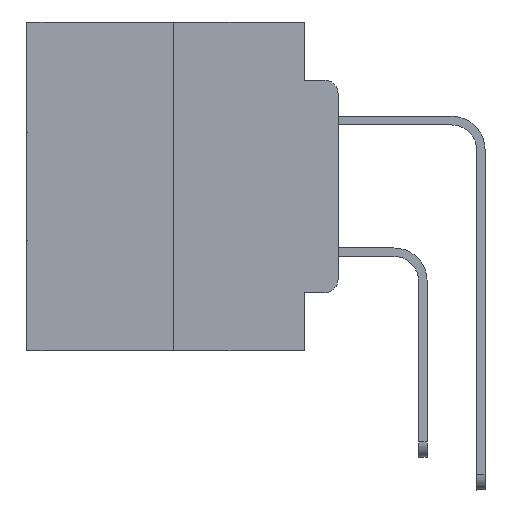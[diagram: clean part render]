
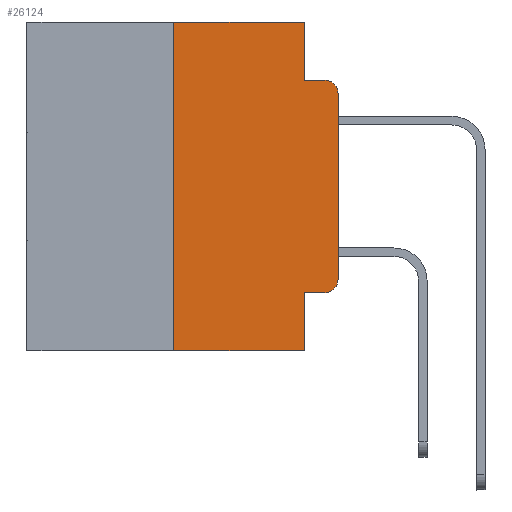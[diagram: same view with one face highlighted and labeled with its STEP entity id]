
A CAD part, left-side view. The second image highlights one B-rep face of the part: STEP entity #26124.
In plain terms, the highlighted planar face has unit normal (-1, 0, 0).
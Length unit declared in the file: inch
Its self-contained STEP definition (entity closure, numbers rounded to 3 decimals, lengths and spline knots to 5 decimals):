
#1481 = EDGE_CURVE ( 'NONE', #4113, #3315, #22992, .T. ) ;
#1578 = LINE ( 'NONE', #7016, #3726 ) ;
#1732 = DIRECTION ( 'NONE',  ( 1., 0., 0. ) ) ;
#2211 = VERTEX_POINT ( 'NONE', #15602 ) ;
#3315 = VERTEX_POINT ( 'NONE', #21942 ) ;
#3334 = ORIENTED_EDGE ( 'NONE', *, *, #27050, .T. ) ;
#3726 = VECTOR ( 'NONE', #4649, 39.37008 ) ;
#4071 = VECTOR ( 'NONE', #12313, 39.37008 ) ;
#4113 = VERTEX_POINT ( 'NONE', #10780 ) ;
#4649 = DIRECTION ( 'NONE',  ( 0., -1., 0. ) ) ;
#5080 = EDGE_CURVE ( 'NONE', #3315, #6023, #9863, .T. ) ;
#5183 = DIRECTION ( 'NONE',  ( -1., 0., 0. ) ) ;
#5289 = VERTEX_POINT ( 'NONE', #11602 ) ;
#6023 = VERTEX_POINT ( 'NONE', #20950 ) ;
#6051 = VERTEX_POINT ( 'NONE', #8245 ) ;
#6160 = PLANE ( 'NONE',  #24197 ) ;
#6342 = CARTESIAN_POINT ( 'NONE',  ( 0., 0.02, -0.0885 ) ) ;
#7016 = CARTESIAN_POINT ( 'NONE',  ( 0., 0.051, -0.0885 ) ) ;
#7912 = ORIENTED_EDGE ( 'NONE', *, *, #14384, .F. ) ;
#8245 = CARTESIAN_POINT ( 'NONE',  ( 0., 0.051, -0.0885 ) ) ;
#8516 = CIRCLE ( 'NONE', #20065, 0.02 ) ;
#8727 = DIRECTION ( 'NONE',  ( 0., 0., -1. ) ) ;
#8908 = VERTEX_POINT ( 'NONE', #6342 ) ;
#9093 = VECTOR ( 'NONE', #23812, 39.37008 ) ;
#9863 = LINE ( 'NONE', #16541, #20151 ) ;
#10456 = LINE ( 'NONE', #21696, #9093 ) ;
#10651 = EDGE_CURVE ( 'NONE', #5289, #26768, #10456, .T. ) ;
#10665 = ORIENTED_EDGE ( 'NONE', *, *, #1481, .T. ) ;
#10780 = CARTESIAN_POINT ( 'NONE',  ( 0., 0.02, -0.4115 ) ) ;
#11130 = AXIS2_PLACEMENT_3D ( 'NONE', #11958, #11979, #24126 ) ;
#11602 = CARTESIAN_POINT ( 'NONE',  ( 0., 0.25, -0.5 ) ) ;
#11958 = CARTESIAN_POINT ( 'NONE',  ( 0., 0.02, -0.3915 ) ) ;
#11979 = DIRECTION ( 'NONE',  ( -1., 0., 0. ) ) ;
#12313 = DIRECTION ( 'NONE',  ( 0., 0., -1. ) ) ;
#12425 = ORIENTED_EDGE ( 'NONE', *, *, #5080, .T. ) ;
#12556 = EDGE_CURVE ( 'NONE', #6051, #8908, #1578, .T. ) ;
#12796 = CARTESIAN_POINT ( 'NONE',  ( 0., 0.473, 0. ) ) ;
#12957 = CARTESIAN_POINT ( 'NONE',  ( 0., 0.051, -0.5 ) ) ;
#13675 = CARTESIAN_POINT ( 'NONE',  ( 0., 0.051, -0.4115 ) ) ;
#14384 = EDGE_CURVE ( 'NONE', #2211, #26014, #16190, .T. ) ;
#15510 = EDGE_CURVE ( 'NONE', #6023, #8908, #8516, .T. ) ;
#15602 = CARTESIAN_POINT ( 'NONE',  ( 0., 0.25, 0. ) ) ;
#15871 = ORIENTED_EDGE ( 'NONE', *, *, #24171, .F. ) ;
#16190 = LINE ( 'NONE', #26641, #19915 ) ;
#16541 = CARTESIAN_POINT ( 'NONE',  ( 0., 0., 0. ) ) ;
#17233 = ORIENTED_EDGE ( 'NONE', *, *, #18422, .F. ) ;
#17292 = DIRECTION ( 'NONE',  ( 0., 0., -1. ) ) ;
#18422 = EDGE_CURVE ( 'NONE', #26014, #6051, #27694, .T. ) ;
#18427 = CARTESIAN_POINT ( 'NONE',  ( 0., 0.02, -0.1085 ) ) ;
#18756 = VECTOR ( 'NONE', #23254, 39.37008 ) ;
#18913 = ORIENTED_EDGE ( 'NONE', *, *, #12556, .F. ) ;
#18998 = CARTESIAN_POINT ( 'NONE',  ( 0., 0.051, 0. ) ) ;
#19189 = DIRECTION ( 'NONE',  ( 0., -1., 0. ) ) ;
#19423 = LINE ( 'NONE', #21117, #18756 ) ;
#19592 = ORIENTED_EDGE ( 'NONE', *, *, #21337, .F. ) ;
#19665 = CARTESIAN_POINT ( 'NONE',  ( 0., 0.051, 0. ) ) ;
#19915 = VECTOR ( 'NONE', #22370, 39.37008 ) ;
#20065 = AXIS2_PLACEMENT_3D ( 'NONE', #18427, #5183, #20606 ) ;
#20151 = VECTOR ( 'NONE', #27908, 39.37008 ) ;
#20280 = ORIENTED_EDGE ( 'NONE', *, *, #10651, .T. ) ;
#20606 = DIRECTION ( 'NONE',  ( 0., 0., -1. ) ) ;
#20950 = CARTESIAN_POINT ( 'NONE',  ( 0., 0., -0.1085 ) ) ;
#21075 = EDGE_LOOP ( 'NONE', ( #12425, #23956, #18913, #17233, #7912, #19592, #20280, #15871, #3334, #10665 ) ) ;
#21117 = CARTESIAN_POINT ( 'NONE',  ( 0., 0.25, 0. ) ) ;
#21337 = EDGE_CURVE ( 'NONE', #5289, #2211, #19423, .T. ) ;
#21696 = CARTESIAN_POINT ( 'NONE',  ( 0., 0.473, -0.5 ) ) ;
#21706 = VERTEX_POINT ( 'NONE', #13675 ) ;
#21942 = CARTESIAN_POINT ( 'NONE',  ( 0., 0., -0.3915 ) ) ;
#22058 = VECTOR ( 'NONE', #8727, 39.37008 ) ;
#22370 = DIRECTION ( 'NONE',  ( 0., -1., 0. ) ) ;
#22992 = CIRCLE ( 'NONE', #11130, 0.02 ) ;
#23254 = DIRECTION ( 'NONE',  ( 0., 0., 1. ) ) ;
#23756 = LINE ( 'NONE', #27798, #28077 ) ;
#23812 = DIRECTION ( 'NONE',  ( 0., -1., 0. ) ) ;
#23956 = ORIENTED_EDGE ( 'NONE', *, *, #15510, .T. ) ;
#24126 = DIRECTION ( 'NONE',  ( 0., 0., -1. ) ) ;
#24171 = EDGE_CURVE ( 'NONE', #21706, #26768, #24634, .T. ) ;
#24197 = AXIS2_PLACEMENT_3D ( 'NONE', #12796, #1732, #17292 ) ;
#24634 = LINE ( 'NONE', #25258, #4071 ) ;
#25258 = CARTESIAN_POINT ( 'NONE',  ( 0., 0.051, 0. ) ) ;
#25883 = FACE_OUTER_BOUND ( 'NONE', #21075, .T. ) ;
#26014 = VERTEX_POINT ( 'NONE', #18998 ) ;
#26124 = ADVANCED_FACE ( 'NONE', ( #25883 ), #6160, .F. ) ;
#26641 = CARTESIAN_POINT ( 'NONE',  ( 0., 0.473, 0. ) ) ;
#26768 = VERTEX_POINT ( 'NONE', #12957 ) ;
#27050 = EDGE_CURVE ( 'NONE', #21706, #4113, #23756, .T. ) ;
#27694 = LINE ( 'NONE', #19665, #22058 ) ;
#27798 = CARTESIAN_POINT ( 'NONE',  ( 0., 0.051, -0.4115 ) ) ;
#27908 = DIRECTION ( 'NONE',  ( 0., 0., 1. ) ) ;
#28077 = VECTOR ( 'NONE', #19189, 39.37008 ) ;
